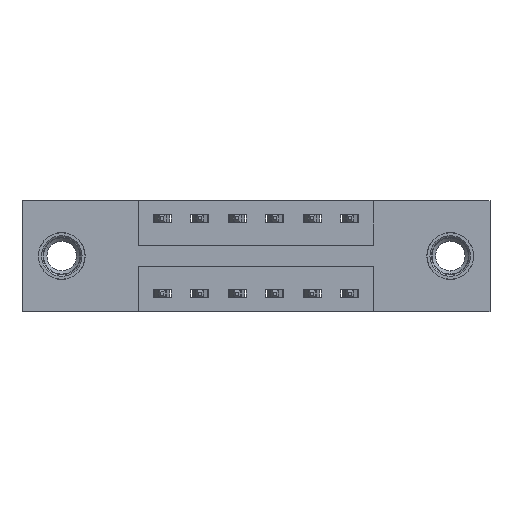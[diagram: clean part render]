
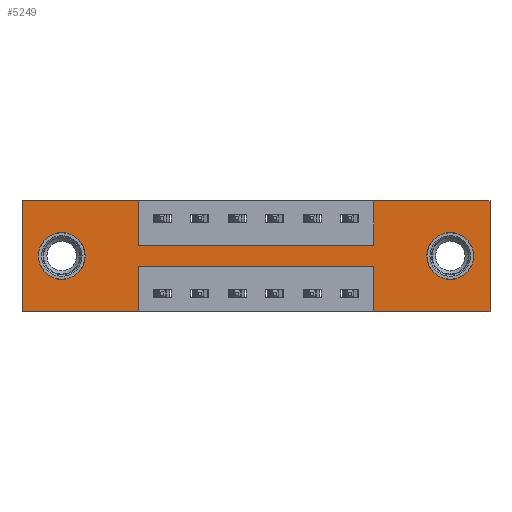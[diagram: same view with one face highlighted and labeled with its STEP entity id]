
A CAD part, front view. The second image highlights one B-rep face of the part: STEP entity #5249.
In plain terms, the highlighted planar face has unit normal (0, -1, 0).
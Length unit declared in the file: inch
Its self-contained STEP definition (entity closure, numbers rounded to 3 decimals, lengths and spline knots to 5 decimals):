
#14 = CARTESIAN_POINT ( 'NONE',  ( 0., 0., 0. ) ) ;
#34 = DIRECTION ( 'NONE',  ( 0., 0., -1. ) ) ;
#68 = EDGE_CURVE ( 'NONE', #8466, #4305, #3234, .T. ) ;
#106 = CARTESIAN_POINT ( 'NONE',  ( 0., 0., -0.37 ) ) ;
#248 = VERTEX_POINT ( 'NONE', #6909 ) ;
#328 = CARTESIAN_POINT ( 'NONE',  ( 1.1725, 0., -0.37 ) ) ;
#332 = EDGE_LOOP ( 'NONE', ( #410, #5076 ) ) ;
#410 = ORIENTED_EDGE ( 'NONE', *, *, #3213, .T. ) ;
#436 = VERTEX_POINT ( 'NONE', #5988 ) ;
#440 = CARTESIAN_POINT ( 'NONE',  ( 0.1325, 0., -0.107 ) ) ;
#485 = VERTEX_POINT ( 'NONE', #3756 ) ;
#529 = ORIENTED_EDGE ( 'NONE', *, *, #9030, .F. ) ;
#549 = VERTEX_POINT ( 'NONE', #440 ) ;
#590 = CARTESIAN_POINT ( 'NONE',  ( 0.3875, 0., -0.37 ) ) ;
#643 = CIRCLE ( 'NONE', #4802, 0.078 ) ;
#769 = CIRCLE ( 'NONE', #3946, 0.078 ) ;
#945 = VECTOR ( 'NONE', #7537, 39.37008 ) ;
#1056 = VECTOR ( 'NONE', #6244, 39.37008 ) ;
#1104 = CARTESIAN_POINT ( 'NONE',  ( 1.4275, 0., -0.185 ) ) ;
#1163 = CARTESIAN_POINT ( 'NONE',  ( 1.1725, 0., 0. ) ) ;
#1312 = FACE_BOUND ( 'NONE', #6171, .T. ) ;
#1421 = ORIENTED_EDGE ( 'NONE', *, *, #4993, .T. ) ;
#1531 = VECTOR ( 'NONE', #4667, 39.37008 ) ;
#1532 = VERTEX_POINT ( 'NONE', #1739 ) ;
#1571 = CARTESIAN_POINT ( 'NONE',  ( 0., 0., 0. ) ) ;
#1589 = CARTESIAN_POINT ( 'NONE',  ( 0.3875, 0., -0.15 ) ) ;
#1624 = EDGE_CURVE ( 'NONE', #436, #1532, #3354, .T. ) ;
#1673 = EDGE_CURVE ( 'NONE', #4305, #8227, #8490, .T. ) ;
#1702 = PLANE ( 'NONE',  #4505 ) ;
#1739 = CARTESIAN_POINT ( 'NONE',  ( 1.1725, 0., -0.22 ) ) ;
#1798 = VERTEX_POINT ( 'NONE', #8234 ) ;
#1882 = DIRECTION ( 'NONE',  ( 0., 1., 0. ) ) ;
#1916 = EDGE_CURVE ( 'NONE', #5033, #248, #4924, .T. ) ;
#1942 = EDGE_CURVE ( 'NONE', #1532, #3019, #5168, .T. ) ;
#2043 = LINE ( 'NONE', #4546, #2286 ) ;
#2113 = CIRCLE ( 'NONE', #7237, 0.078 ) ;
#2228 = CARTESIAN_POINT ( 'NONE',  ( 0.3875, 0., -0.22 ) ) ;
#2270 = CARTESIAN_POINT ( 'NONE',  ( 0., 0., 0. ) ) ;
#2275 = CARTESIAN_POINT ( 'NONE',  ( 0.1325, 0., -0.185 ) ) ;
#2286 = VECTOR ( 'NONE', #8415, 39.37008 ) ;
#2310 = DIRECTION ( 'NONE',  ( 0., 0., 1. ) ) ;
#2400 = CARTESIAN_POINT ( 'NONE',  ( 0., 0., 0. ) ) ;
#2505 = DIRECTION ( 'NONE',  ( 0., 1., 0. ) ) ;
#2543 = ORIENTED_EDGE ( 'NONE', *, *, #2636, .F. ) ;
#2636 = EDGE_CURVE ( 'NONE', #485, #5033, #5015, .T. ) ;
#2771 = AXIS2_PLACEMENT_3D ( 'NONE', #1104, #6678, #9767 ) ;
#2804 = DIRECTION ( 'NONE',  ( 0., 0., 1. ) ) ;
#2845 = LINE ( 'NONE', #2270, #6451 ) ;
#2849 = CARTESIAN_POINT ( 'NONE',  ( 0.3875, 0., -0.15 ) ) ;
#2853 = EDGE_CURVE ( 'NONE', #3366, #549, #2113, .T. ) ;
#3019 = VERTEX_POINT ( 'NONE', #4843 ) ;
#3087 = VECTOR ( 'NONE', #7643, 39.37008 ) ;
#3102 = CARTESIAN_POINT ( 'NONE',  ( 0., 0., -0.37 ) ) ;
#3213 = EDGE_CURVE ( 'NONE', #549, #3366, #643, .T. ) ;
#3234 = LINE ( 'NONE', #14, #1056 ) ;
#3243 = ORIENTED_EDGE ( 'NONE', *, *, #8989, .F. ) ;
#3276 = DIRECTION ( 'NONE',  ( 0., 0., 1. ) ) ;
#3354 = LINE ( 'NONE', #328, #6843 ) ;
#3364 = EDGE_CURVE ( 'NONE', #9256, #3615, #6788, .T. ) ;
#3366 = VERTEX_POINT ( 'NONE', #4716 ) ;
#3615 = VERTEX_POINT ( 'NONE', #2400 ) ;
#3756 = CARTESIAN_POINT ( 'NONE',  ( 0.3875, 0., 0. ) ) ;
#3834 = FACE_OUTER_BOUND ( 'NONE', #7914, .T. ) ;
#3946 = AXIS2_PLACEMENT_3D ( 'NONE', #5695, #1882, #7962 ) ;
#3953 = VERTEX_POINT ( 'NONE', #4491 ) ;
#4232 = DIRECTION ( 'NONE',  ( 0., 0., -1. ) ) ;
#4305 = VERTEX_POINT ( 'NONE', #6258 ) ;
#4491 = CARTESIAN_POINT ( 'NONE',  ( 1.4275, 0., -0.263 ) ) ;
#4505 = AXIS2_PLACEMENT_3D ( 'NONE', #106, #8581, #34 ) ;
#4546 = CARTESIAN_POINT ( 'NONE',  ( 0., 0., -0.37 ) ) ;
#4557 = EDGE_CURVE ( 'NONE', #248, #8466, #6643, .T. ) ;
#4601 = DIRECTION ( 'NONE',  ( 0., 0., 1. ) ) ;
#4667 = DIRECTION ( 'NONE',  ( 1., 0., 0. ) ) ;
#4716 = CARTESIAN_POINT ( 'NONE',  ( 0.1325, 0., -0.263 ) ) ;
#4802 = AXIS2_PLACEMENT_3D ( 'NONE', #4818, #2505, #3276 ) ;
#4818 = CARTESIAN_POINT ( 'NONE',  ( 0.1325, 0., -0.185 ) ) ;
#4837 = CARTESIAN_POINT ( 'NONE',  ( 1.4275, 0., -0.107 ) ) ;
#4843 = CARTESIAN_POINT ( 'NONE',  ( 0.3875, 0., -0.22 ) ) ;
#4924 = LINE ( 'NONE', #1589, #1531 ) ;
#4956 = DIRECTION ( 'NONE',  ( 0., 0., -1. ) ) ;
#4969 = FACE_BOUND ( 'NONE', #332, .T. ) ;
#4993 = EDGE_CURVE ( 'NONE', #3953, #7619, #5911, .T. ) ;
#5015 = LINE ( 'NONE', #7993, #8005 ) ;
#5033 = VERTEX_POINT ( 'NONE', #2849 ) ;
#5076 = ORIENTED_EDGE ( 'NONE', *, *, #2853, .T. ) ;
#5168 = LINE ( 'NONE', #2228, #3087 ) ;
#5249 = ADVANCED_FACE ( 'NONE', ( #1312, #4969, #3834 ), #1702, .T. ) ;
#5467 = ORIENTED_EDGE ( 'NONE', *, *, #1673, .F. ) ;
#5659 = EDGE_CURVE ( 'NONE', #1798, #9256, #2043, .T. ) ;
#5695 = CARTESIAN_POINT ( 'NONE',  ( 1.4275, 0., -0.185 ) ) ;
#5911 = CIRCLE ( 'NONE', #2771, 0.078 ) ;
#5988 = CARTESIAN_POINT ( 'NONE',  ( 1.1725, 0., -0.37 ) ) ;
#6007 = ORIENTED_EDGE ( 'NONE', *, *, #9580, .T. ) ;
#6109 = LINE ( 'NONE', #590, #945 ) ;
#6168 = EDGE_CURVE ( 'NONE', #3019, #1798, #6109, .T. ) ;
#6171 = EDGE_LOOP ( 'NONE', ( #6007, #1421 ) ) ;
#6244 = DIRECTION ( 'NONE',  ( 1., 0., 0. ) ) ;
#6258 = CARTESIAN_POINT ( 'NONE',  ( 1.56, 0., 0. ) ) ;
#6329 = ORIENTED_EDGE ( 'NONE', *, *, #1916, .F. ) ;
#6450 = VECTOR ( 'NONE', #4232, 39.37008 ) ;
#6451 = VECTOR ( 'NONE', #9923, 39.37008 ) ;
#6560 = LINE ( 'NONE', #3102, #9082 ) ;
#6643 = LINE ( 'NONE', #8074, #9530 ) ;
#6678 = DIRECTION ( 'NONE',  ( 0., 1., 0. ) ) ;
#6788 = LINE ( 'NONE', #1571, #7155 ) ;
#6813 = CARTESIAN_POINT ( 'NONE',  ( 1.56, 0., -0.37 ) ) ;
#6843 = VECTOR ( 'NONE', #8799, 39.37008 ) ;
#6866 = ORIENTED_EDGE ( 'NONE', *, *, #6168, .F. ) ;
#6909 = CARTESIAN_POINT ( 'NONE',  ( 1.1725, 0., -0.15 ) ) ;
#7155 = VECTOR ( 'NONE', #4601, 39.37008 ) ;
#7237 = AXIS2_PLACEMENT_3D ( 'NONE', #2275, #9153, #2310 ) ;
#7409 = ORIENTED_EDGE ( 'NONE', *, *, #1942, .F. ) ;
#7410 = ORIENTED_EDGE ( 'NONE', *, *, #3364, .F. ) ;
#7537 = DIRECTION ( 'NONE',  ( 0., 0., -1. ) ) ;
#7557 = CARTESIAN_POINT ( 'NONE',  ( 0., 0., -0.37 ) ) ;
#7619 = VERTEX_POINT ( 'NONE', #4837 ) ;
#7643 = DIRECTION ( 'NONE',  ( -1., 0., 0. ) ) ;
#7914 = EDGE_LOOP ( 'NONE', ( #6866, #7409, #8211, #529, #5467, #8259, #9536, #6329, #2543, #3243, #7410, #8858 ) ) ;
#7962 = DIRECTION ( 'NONE',  ( 0., 0., -1. ) ) ;
#7993 = CARTESIAN_POINT ( 'NONE',  ( 0.3875, 0., 0. ) ) ;
#8005 = VECTOR ( 'NONE', #4956, 39.37008 ) ;
#8074 = CARTESIAN_POINT ( 'NONE',  ( 1.1725, 0., 0. ) ) ;
#8081 = CARTESIAN_POINT ( 'NONE',  ( 1.56, 0., 0. ) ) ;
#8211 = ORIENTED_EDGE ( 'NONE', *, *, #1624, .F. ) ;
#8227 = VERTEX_POINT ( 'NONE', #6813 ) ;
#8234 = CARTESIAN_POINT ( 'NONE',  ( 0.3875, 0., -0.37 ) ) ;
#8259 = ORIENTED_EDGE ( 'NONE', *, *, #68, .F. ) ;
#8415 = DIRECTION ( 'NONE',  ( -1., 0., 0. ) ) ;
#8466 = VERTEX_POINT ( 'NONE', #1163 ) ;
#8490 = LINE ( 'NONE', #8081, #6450 ) ;
#8576 = DIRECTION ( 'NONE',  ( -1., 0., 0. ) ) ;
#8581 = DIRECTION ( 'NONE',  ( 0., -1., 0. ) ) ;
#8799 = DIRECTION ( 'NONE',  ( 0., 0., 1. ) ) ;
#8858 = ORIENTED_EDGE ( 'NONE', *, *, #5659, .F. ) ;
#8989 = EDGE_CURVE ( 'NONE', #3615, #485, #2845, .T. ) ;
#9030 = EDGE_CURVE ( 'NONE', #8227, #436, #6560, .T. ) ;
#9082 = VECTOR ( 'NONE', #8576, 39.37008 ) ;
#9153 = DIRECTION ( 'NONE',  ( 0., 1., 0. ) ) ;
#9256 = VERTEX_POINT ( 'NONE', #7557 ) ;
#9530 = VECTOR ( 'NONE', #2804, 39.37008 ) ;
#9536 = ORIENTED_EDGE ( 'NONE', *, *, #4557, .F. ) ;
#9580 = EDGE_CURVE ( 'NONE', #7619, #3953, #769, .T. ) ;
#9767 = DIRECTION ( 'NONE',  ( 0., 0., -1. ) ) ;
#9923 = DIRECTION ( 'NONE',  ( 1., 0., 0. ) ) ;
